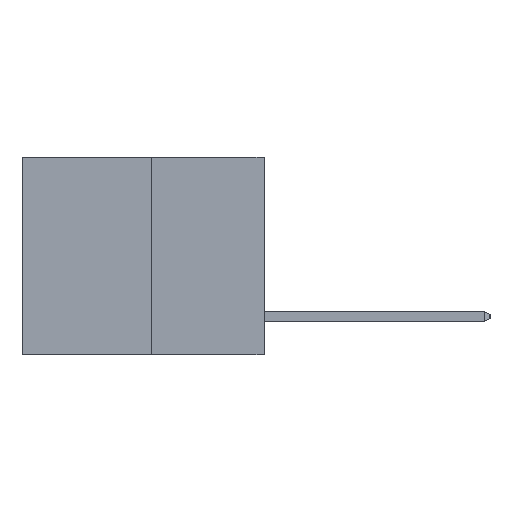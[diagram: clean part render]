
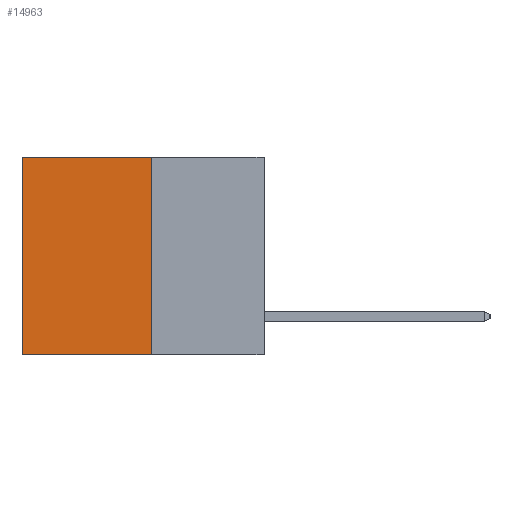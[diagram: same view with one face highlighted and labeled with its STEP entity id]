
A CAD part, left-side view. The second image highlights one B-rep face of the part: STEP entity #14963.
In plain terms, the highlighted planar face has unit normal (-1, 0, 0).
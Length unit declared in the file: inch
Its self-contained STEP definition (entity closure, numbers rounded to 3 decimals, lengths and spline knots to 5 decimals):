
#291 = DIRECTION ( 'NONE',  ( 0., 0., -1. ) ) ;
#1046 = EDGE_LOOP ( 'NONE', ( #14071, #15449, #5918, #25214 ) ) ;
#1460 = AXIS2_PLACEMENT_3D ( 'NONE', #8696, #16793, #291 ) ;
#1771 = CARTESIAN_POINT ( 'NONE',  ( 0.3165, 0.28, 0. ) ) ;
#2075 = EDGE_CURVE ( 'NONE', #5611, #23162, #22976, .T. ) ;
#3483 = EDGE_CURVE ( 'NONE', #12722, #23162, #10519, .T. ) ;
#3645 = CARTESIAN_POINT ( 'NONE',  ( 0.3165, 0.6, 0. ) ) ;
#3964 = VECTOR ( 'NONE', #22591, 39.37008 ) ;
#4532 = CARTESIAN_POINT ( 'NONE',  ( 0.3165, 0.28, -0.49 ) ) ;
#5158 = VECTOR ( 'NONE', #6838, 39.37008 ) ;
#5485 = FACE_OUTER_BOUND ( 'NONE', #1046, .T. ) ;
#5611 = VERTEX_POINT ( 'NONE', #22351 ) ;
#5918 = ORIENTED_EDGE ( 'NONE', *, *, #20071, .F. ) ;
#6838 = DIRECTION ( 'NONE',  ( 0., 0., -1. ) ) ;
#7031 = CARTESIAN_POINT ( 'NONE',  ( 0.3165, 0.28, 0. ) ) ;
#8696 = CARTESIAN_POINT ( 'NONE',  ( 0.3165, 0.28, -0.49 ) ) ;
#8778 = CARTESIAN_POINT ( 'NONE',  ( 0.3165, 0.28, -0.49 ) ) ;
#10519 = LINE ( 'NONE', #20476, #15556 ) ;
#10781 = EDGE_CURVE ( 'NONE', #21960, #12722, #11447, .T. ) ;
#11447 = LINE ( 'NONE', #7031, #15417 ) ;
#12722 = VERTEX_POINT ( 'NONE', #3645 ) ;
#13225 = DIRECTION ( 'NONE',  ( 0., 1., 0. ) ) ;
#14071 = ORIENTED_EDGE ( 'NONE', *, *, #3483, .T. ) ;
#14963 = ADVANCED_FACE ( 'NONE', ( #5485 ), #18782, .F. ) ;
#15417 = VECTOR ( 'NONE', #13225, 39.37008 ) ;
#15449 = ORIENTED_EDGE ( 'NONE', *, *, #2075, .F. ) ;
#15556 = VECTOR ( 'NONE', #16558, 39.37008 ) ;
#16558 = DIRECTION ( 'NONE',  ( 0., 0., -1. ) ) ;
#16793 = DIRECTION ( 'NONE',  ( 1., 0., 0. ) ) ;
#18782 = PLANE ( 'NONE',  #1460 ) ;
#20071 = EDGE_CURVE ( 'NONE', #21960, #5611, #26012, .T. ) ;
#20476 = CARTESIAN_POINT ( 'NONE',  ( 0.3165, 0.6, -0.49 ) ) ;
#21960 = VERTEX_POINT ( 'NONE', #1771 ) ;
#22351 = CARTESIAN_POINT ( 'NONE',  ( 0.3165, 0.28, -0.49 ) ) ;
#22591 = DIRECTION ( 'NONE',  ( 0., 1., 0. ) ) ;
#22976 = LINE ( 'NONE', #8778, #3964 ) ;
#23162 = VERTEX_POINT ( 'NONE', #23886 ) ;
#23886 = CARTESIAN_POINT ( 'NONE',  ( 0.3165, 0.6, -0.49 ) ) ;
#25214 = ORIENTED_EDGE ( 'NONE', *, *, #10781, .T. ) ;
#26012 = LINE ( 'NONE', #4532, #5158 ) ;
